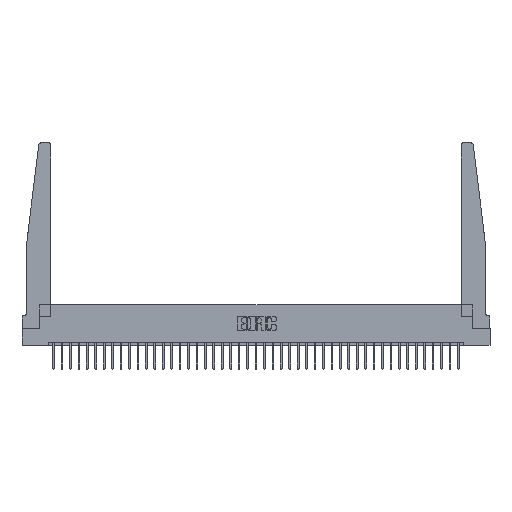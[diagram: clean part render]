
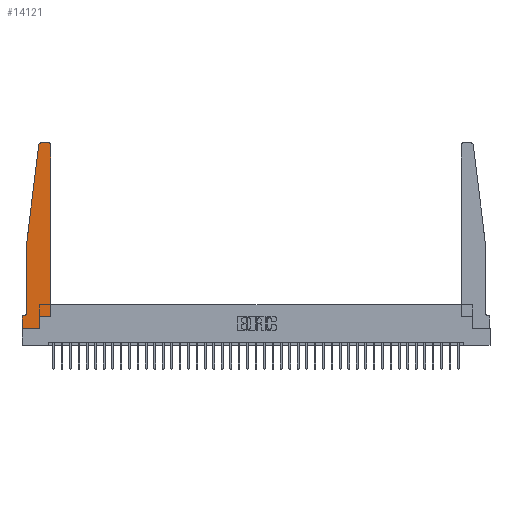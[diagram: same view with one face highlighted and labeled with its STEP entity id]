
A CAD part, top view. The second image highlights one B-rep face of the part: STEP entity #14121.
In plain terms, the highlighted planar face has unit normal (0, 0, 1).
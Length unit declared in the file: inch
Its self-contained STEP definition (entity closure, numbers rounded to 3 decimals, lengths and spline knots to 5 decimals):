
#370 = DIRECTION ( 'NONE',  ( 0., 0., 1. ) ) ;
#697 = VECTOR ( 'NONE', #13289, 39.37008 ) ;
#1221 = CARTESIAN_POINT ( 'NONE',  ( 0.065, 0.1875, 0.37 ) ) ;
#1473 = DIRECTION ( 'NONE',  ( 0., 0., 1. ) ) ;
#1654 = CARTESIAN_POINT ( 'NONE',  ( 0., 0.1875, 0.37 ) ) ;
#1713 = LINE ( 'NONE', #1221, #26386 ) ;
#1754 = EDGE_CURVE ( 'NONE', #16428, #32986, #1713, .T. ) ;
#2009 = ORIENTED_EDGE ( 'NONE', *, *, #30812, .T. ) ;
#2785 = CARTESIAN_POINT ( 'NONE',  ( 0.065, 0.2375, 0.37 ) ) ;
#2879 = LINE ( 'NONE', #25521, #22772 ) ;
#2889 = CARTESIAN_POINT ( 'NONE',  ( 0.2605, 0., 0.37 ) ) ;
#3859 = CIRCLE ( 'NONE', #13695, 0.05 ) ;
#4158 = VERTEX_POINT ( 'NONE', #2889 ) ;
#4626 = VERTEX_POINT ( 'NONE', #34683 ) ;
#4910 = CARTESIAN_POINT ( 'NONE',  ( 0.015, 0.1875, 0.37 ) ) ;
#5304 = EDGE_CURVE ( 'NONE', #26369, #15606, #6595, .T. ) ;
#6059 = CARTESIAN_POINT ( 'NONE',  ( 0.065, 1.25, 0.37 ) ) ;
#6086 = CARTESIAN_POINT ( 'NONE',  ( 0.27653, 2.72, 0.37 ) ) ;
#6588 = LINE ( 'NONE', #6059, #22167 ) ;
#6595 = LINE ( 'NONE', #31134, #22577 ) ;
#7053 = DIRECTION ( 'NONE',  ( 0., 0., -1. ) ) ;
#7174 = CARTESIAN_POINT ( 'NONE',  ( 0.015, 0.2375, 0.37 ) ) ;
#7593 = EDGE_CURVE ( 'NONE', #28773, #4158, #12845, .T. ) ;
#7656 = PLANE ( 'NONE',  #34053 ) ;
#7714 = VECTOR ( 'NONE', #28023, 39.37008 ) ;
#7927 = ORIENTED_EDGE ( 'NONE', *, *, #12000, .T. ) ;
#8410 = CARTESIAN_POINT ( 'NONE',  ( 0., 0., 0.37 ) ) ;
#9039 = CARTESIAN_POINT ( 'NONE',  ( 0., 0., 0.37 ) ) ;
#9347 = CARTESIAN_POINT ( 'NONE',  ( 0.425, 0.18, 0.37 ) ) ;
#9496 = CARTESIAN_POINT ( 'NONE',  ( 0.2605, 0.18, 0.37 ) ) ;
#9784 = EDGE_CURVE ( 'NONE', #25422, #4626, #16279, .T. ) ;
#10311 = ORIENTED_EDGE ( 'NONE', *, *, #31124, .T. ) ;
#10598 = EDGE_CURVE ( 'NONE', #32986, #28773, #32268, .T. ) ;
#11367 = VERTEX_POINT ( 'NONE', #34201 ) ;
#12000 = EDGE_CURVE ( 'NONE', #15606, #32587, #2879, .T. ) ;
#12681 = FACE_OUTER_BOUND ( 'NONE', #23084, .T. ) ;
#12845 = LINE ( 'NONE', #8410, #7714 ) ;
#13032 = CARTESIAN_POINT ( 'NONE',  ( 0.25, 2.75, 0.37 ) ) ;
#13068 = ORIENTED_EDGE ( 'NONE', *, *, #9784, .T. ) ;
#13289 = DIRECTION ( 'NONE',  ( -1., 0., 0. ) ) ;
#13523 = VECTOR ( 'NONE', #13945, 39.37008 ) ;
#13695 = AXIS2_PLACEMENT_3D ( 'NONE', #7174, #7053, #21778 ) ;
#13945 = DIRECTION ( 'NONE',  ( 0., -1., 0. ) ) ;
#14121 = ADVANCED_FACE ( 'NONE', ( #12681 ), #7656, .T. ) ;
#14250 = VECTOR ( 'NONE', #34352, 39.37008 ) ;
#15606 = VERTEX_POINT ( 'NONE', #9347 ) ;
#15818 = CARTESIAN_POINT ( 'NONE',  ( 0., 0., 0.37 ) ) ;
#16214 = VERTEX_POINT ( 'NONE', #22892 ) ;
#16279 = LINE ( 'NONE', #13032, #697 ) ;
#16428 = VERTEX_POINT ( 'NONE', #4910 ) ;
#16491 = DIRECTION ( 'NONE',  ( 1., 0., 0. ) ) ;
#17355 = ORIENTED_EDGE ( 'NONE', *, *, #27392, .T. ) ;
#17517 = DIRECTION ( 'NONE',  ( 1., 0., 0. ) ) ;
#18265 = CARTESIAN_POINT ( 'NONE',  ( 0.395, 2.72, 0.37 ) ) ;
#19722 = CARTESIAN_POINT ( 'NONE',  ( 0.395, 2.75, 0.37 ) ) ;
#19876 = DIRECTION ( 'NONE',  ( 1., 0., 0. ) ) ;
#21344 = LINE ( 'NONE', #30490, #13523 ) ;
#21778 = DIRECTION ( 'NONE',  ( -1., 0., 0. ) ) ;
#21880 = CIRCLE ( 'NONE', #30143, 0.03 ) ;
#22034 = ORIENTED_EDGE ( 'NONE', *, *, #10598, .T. ) ;
#22167 = VECTOR ( 'NONE', #34028, 39.37008 ) ;
#22577 = VECTOR ( 'NONE', #17517, 39.37008 ) ;
#22772 = VECTOR ( 'NONE', #28806, 39.37008 ) ;
#22892 = CARTESIAN_POINT ( 'NONE',  ( 0.065, 1.25, 0.37 ) ) ;
#23084 = EDGE_LOOP ( 'NONE', ( #13068, #2009, #23171, #17355, #10311, #33212, #22034, #24538, #25284, #31145, #7927, #32116 ) ) ;
#23171 = ORIENTED_EDGE ( 'NONE', *, *, #27923, .T. ) ;
#23438 = AXIS2_PLACEMENT_3D ( 'NONE', #6086, #25570, #19876 ) ;
#24538 = ORIENTED_EDGE ( 'NONE', *, *, #7593, .T. ) ;
#24880 = VECTOR ( 'NONE', #31018, 39.37008 ) ;
#25284 = ORIENTED_EDGE ( 'NONE', *, *, #30278, .T. ) ;
#25422 = VERTEX_POINT ( 'NONE', #19722 ) ;
#25521 = CARTESIAN_POINT ( 'NONE',  ( 0.425, 0.18, 0.37 ) ) ;
#25570 = DIRECTION ( 'NONE',  ( 0., 0., 1. ) ) ;
#25712 = EDGE_CURVE ( 'NONE', #32587, #25422, #21880, .T. ) ;
#26369 = VERTEX_POINT ( 'NONE', #34761 ) ;
#26386 = VECTOR ( 'NONE', #28030, 39.37008 ) ;
#27392 = EDGE_CURVE ( 'NONE', #16214, #30040, #21344, .T. ) ;
#27923 = EDGE_CURVE ( 'NONE', #11367, #16214, #6588, .T. ) ;
#28023 = DIRECTION ( 'NONE',  ( 1., 0., 0. ) ) ;
#28030 = DIRECTION ( 'NONE',  ( -1., 0., 0. ) ) ;
#28773 = VERTEX_POINT ( 'NONE', #9039 ) ;
#28806 = DIRECTION ( 'NONE',  ( 0., 1., 0. ) ) ;
#30040 = VERTEX_POINT ( 'NONE', #2785 ) ;
#30143 = AXIS2_PLACEMENT_3D ( 'NONE', #18265, #1473, #34390 ) ;
#30278 = EDGE_CURVE ( 'NONE', #4158, #26369, #32910, .T. ) ;
#30490 = CARTESIAN_POINT ( 'NONE',  ( 0.065, 1.25, 0.37 ) ) ;
#30812 = EDGE_CURVE ( 'NONE', #4626, #11367, #31172, .T. ) ;
#31018 = DIRECTION ( 'NONE',  ( 0., -1., 0. ) ) ;
#31124 = EDGE_CURVE ( 'NONE', #30040, #16428, #3859, .T. ) ;
#31134 = CARTESIAN_POINT ( 'NONE',  ( 0.425, 0.18, 0.37 ) ) ;
#31145 = ORIENTED_EDGE ( 'NONE', *, *, #5304, .T. ) ;
#31172 = CIRCLE ( 'NONE', #23438, 0.03 ) ;
#32116 = ORIENTED_EDGE ( 'NONE', *, *, #25712, .T. ) ;
#32268 = LINE ( 'NONE', #15818, #24880 ) ;
#32587 = VERTEX_POINT ( 'NONE', #33585 ) ;
#32602 = CARTESIAN_POINT ( 'NONE',  ( 0., 0.1875, 0.37 ) ) ;
#32910 = LINE ( 'NONE', #9496, #14250 ) ;
#32986 = VERTEX_POINT ( 'NONE', #1654 ) ;
#33212 = ORIENTED_EDGE ( 'NONE', *, *, #1754, .T. ) ;
#33585 = CARTESIAN_POINT ( 'NONE',  ( 0.425, 2.72, 0.37 ) ) ;
#34028 = DIRECTION ( 'NONE',  ( -0.122, -0.992, 0. ) ) ;
#34053 = AXIS2_PLACEMENT_3D ( 'NONE', #32602, #370, #16491 ) ;
#34201 = CARTESIAN_POINT ( 'NONE',  ( 0.24675, 2.72367, 0.37 ) ) ;
#34352 = DIRECTION ( 'NONE',  ( 0., 1., 0. ) ) ;
#34390 = DIRECTION ( 'NONE',  ( 1., 0., 0. ) ) ;
#34683 = CARTESIAN_POINT ( 'NONE',  ( 0.27653, 2.75, 0.37 ) ) ;
#34761 = CARTESIAN_POINT ( 'NONE',  ( 0.2605, 0.18, 0.37 ) ) ;
